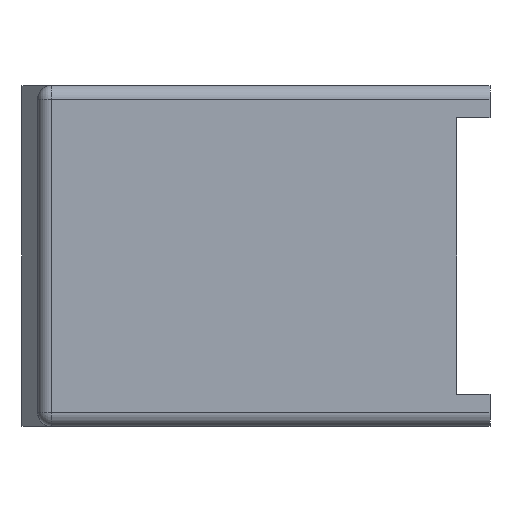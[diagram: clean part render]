
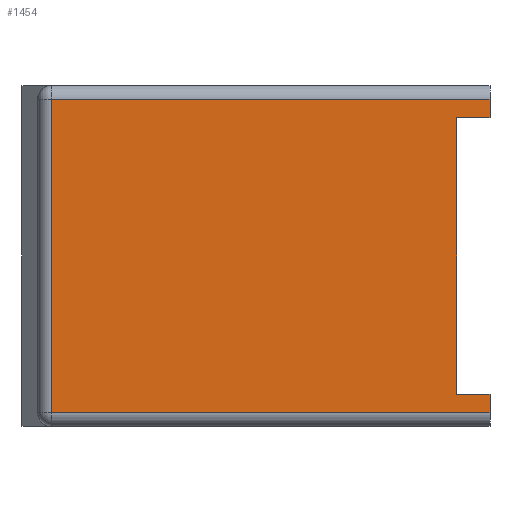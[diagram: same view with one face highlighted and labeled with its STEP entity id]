
A CAD part, left-side view. The second image highlights one B-rep face of the part: STEP entity #1454.
In plain terms, the highlighted planar face has unit normal (-1, 0, 0).
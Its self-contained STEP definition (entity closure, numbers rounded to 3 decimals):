
#22 = EDGE_CURVE ( 'NONE', #1540, #666, #1255, .T. ) ;
#58 = DIRECTION ( 'NONE',  ( 0., -1., 0. ) ) ;
#115 = VERTEX_POINT ( 'NONE', #690 ) ;
#135 = EDGE_LOOP ( 'NONE', ( #2475, #2437, #2165, #542, #1075, #1524, #1911, #1317 ) ) ;
#178 = VERTEX_POINT ( 'NONE', #1862 ) ;
#210 = VECTOR ( 'NONE', #2083, 1000. ) ;
#213 = CARTESIAN_POINT ( 'NONE',  ( 0., 49.987, -1.575 ) ) ;
#254 = EDGE_CURVE ( 'NONE', #178, #115, #1292, .T. ) ;
#300 = EDGE_CURVE ( 'NONE', #349, #178, #2217, .T. ) ;
#349 = VERTEX_POINT ( 'NONE', #1008 ) ;
#360 = AXIS2_PLACEMENT_3D ( 'NONE', #785, #1370, #2327 ) ;
#404 = VERTEX_POINT ( 'NONE', #1788 ) ;
#433 = DIRECTION ( 'NONE',  ( 0., 0., 1. ) ) ;
#447 = DIRECTION ( 'NONE',  ( 0., 1., 0. ) ) ;
#477 = VERTEX_POINT ( 'NONE', #1422 ) ;
#494 = CARTESIAN_POINT ( 'NONE',  ( 0., 51.562, -1.575 ) ) ;
#542 = ORIENTED_EDGE ( 'NONE', *, *, #254, .F. ) ;
#574 = CARTESIAN_POINT ( 'NONE',  ( 0., 49.987, -37.287 ) ) ;
#589 = DIRECTION ( 'NONE',  ( 0., 0., -1. ) ) ;
#666 = VERTEX_POINT ( 'NONE', #574 ) ;
#678 = VECTOR ( 'NONE', #447, 1000. ) ;
#690 = CARTESIAN_POINT ( 'NONE',  ( 0., 0., -35.179 ) ) ;
#724 = VECTOR ( 'NONE', #1568, 1000. ) ;
#760 = PLANE ( 'NONE',  #360 ) ;
#785 = CARTESIAN_POINT ( 'NONE',  ( 0., 0., -38.862 ) ) ;
#806 = LINE ( 'NONE', #1592, #724 ) ;
#826 = CARTESIAN_POINT ( 'NONE',  ( 0., 0., -37.287 ) ) ;
#959 = EDGE_CURVE ( 'NONE', #477, #115, #1401, .T. ) ;
#989 = CARTESIAN_POINT ( 'NONE',  ( 0., 0., -38.862 ) ) ;
#1008 = CARTESIAN_POINT ( 'NONE',  ( 0., 3.81, -3.683 ) ) ;
#1044 = DIRECTION ( 'NONE',  ( 0., 0., -1. ) ) ;
#1059 = CARTESIAN_POINT ( 'NONE',  ( 0., 0., -1.575 ) ) ;
#1075 = ORIENTED_EDGE ( 'NONE', *, *, #300, .F. ) ;
#1202 = CARTESIAN_POINT ( 'NONE',  ( 0., 3.81, -3.683 ) ) ;
#1215 = LINE ( 'NONE', #1202, #678 ) ;
#1255 = LINE ( 'NONE', #2396, #2219 ) ;
#1292 = LINE ( 'NONE', #1535, #1807 ) ;
#1307 = LINE ( 'NONE', #494, #210 ) ;
#1317 = ORIENTED_EDGE ( 'NONE', *, *, #2008, .T. ) ;
#1370 = DIRECTION ( 'NONE',  ( -1., 0., 0. ) ) ;
#1401 = LINE ( 'NONE', #989, #2368 ) ;
#1422 = CARTESIAN_POINT ( 'NONE',  ( 0., 0., -37.287 ) ) ;
#1454 = ADVANCED_FACE ( 'NONE', ( #1555 ), #760, .T. ) ;
#1524 = ORIENTED_EDGE ( 'NONE', *, *, #1643, .F. ) ;
#1535 = CARTESIAN_POINT ( 'NONE',  ( 0., 3.81, -35.179 ) ) ;
#1540 = VERTEX_POINT ( 'NONE', #213 ) ;
#1555 = FACE_OUTER_BOUND ( 'NONE', #135, .T. ) ;
#1566 = EDGE_CURVE ( 'NONE', #404, #2299, #806, .T. ) ;
#1568 = DIRECTION ( 'NONE',  ( 0., 0., 1. ) ) ;
#1577 = VECTOR ( 'NONE', #1044, 1000. ) ;
#1592 = CARTESIAN_POINT ( 'NONE',  ( 0., 0., -38.862 ) ) ;
#1601 = EDGE_CURVE ( 'NONE', #666, #477, #1912, .T. ) ;
#1643 = EDGE_CURVE ( 'NONE', #404, #349, #1215, .T. ) ;
#1788 = CARTESIAN_POINT ( 'NONE',  ( 0., 0., -3.683 ) ) ;
#1807 = VECTOR ( 'NONE', #2118, 1000. ) ;
#1862 = CARTESIAN_POINT ( 'NONE',  ( 0., 3.81, -35.179 ) ) ;
#1911 = ORIENTED_EDGE ( 'NONE', *, *, #1566, .T. ) ;
#1912 = LINE ( 'NONE', #826, #1978 ) ;
#1978 = VECTOR ( 'NONE', #58, 1000. ) ;
#2008 = EDGE_CURVE ( 'NONE', #2299, #1540, #1307, .T. ) ;
#2083 = DIRECTION ( 'NONE',  ( 0., 1., 0. ) ) ;
#2118 = DIRECTION ( 'NONE',  ( 0., -1., 0. ) ) ;
#2165 = ORIENTED_EDGE ( 'NONE', *, *, #959, .T. ) ;
#2217 = LINE ( 'NONE', #2405, #1577 ) ;
#2219 = VECTOR ( 'NONE', #589, 1000. ) ;
#2299 = VERTEX_POINT ( 'NONE', #1059 ) ;
#2327 = DIRECTION ( 'NONE',  ( 0., 0., 1. ) ) ;
#2368 = VECTOR ( 'NONE', #433, 1000. ) ;
#2396 = CARTESIAN_POINT ( 'NONE',  ( 0., 49.987, -38.862 ) ) ;
#2405 = CARTESIAN_POINT ( 'NONE',  ( 0., 3.81, -35.179 ) ) ;
#2437 = ORIENTED_EDGE ( 'NONE', *, *, #1601, .T. ) ;
#2475 = ORIENTED_EDGE ( 'NONE', *, *, #22, .T. ) ;
